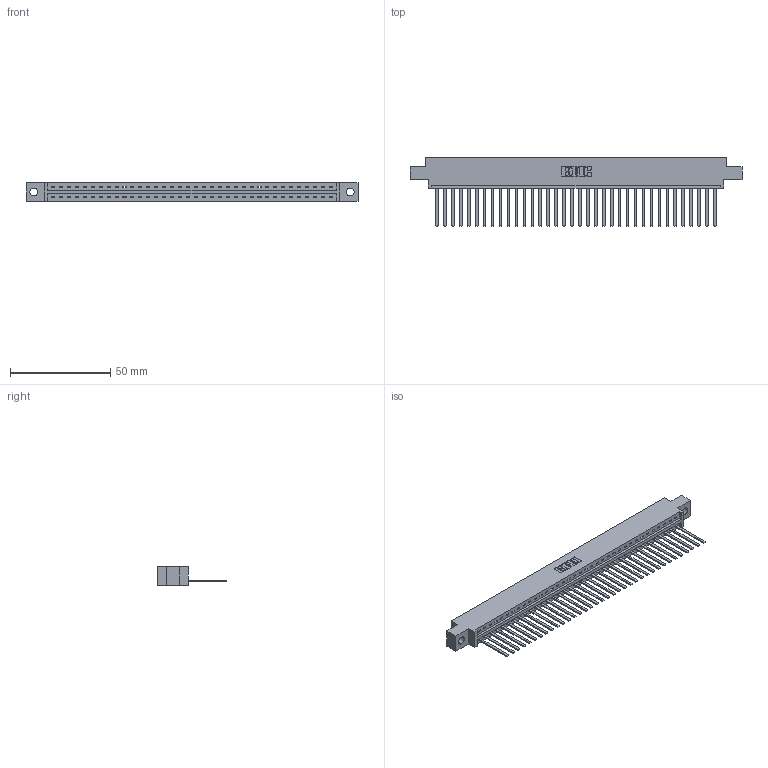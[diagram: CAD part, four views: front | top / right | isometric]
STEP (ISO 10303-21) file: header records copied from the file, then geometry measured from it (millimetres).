
FILE_DESCRIPTION (( 'STEP AP203' ), '1' );
FILE_NAME ('337-036-544-604.STEP', '2018-08-07T23:34:09', ( '' ), ( '' ), 'SwSTEP 2.0', 'SolidWorks 2016', '' );
FILE_SCHEMA (( 'CONFIG_CONTROL_DESIGN' ));
Length unit declared in the file: inch
Products named in the file (3): 345-292-001_345-293-144; 337-036-544-604; 337 Part_0.170 Offset - 0.156 Dia-TH
Assembly tree (37 placements, depth 2):
  337-036-544-604
    337 Part_0.170 Offset - 0.156 Dia-TH
    345-292-001_345-293-144  x36
Bounding box: 165.66 x 34.3 x 9.4 mm (x, y, z)
Volume: 17353.9 mm3; surface area: 19162.6 mm2
Topology: 37 solids, 37 shells, 2134 faces, 6443 edges, 4246 vertices
Faces by surface type: plane 1586, cylinder 548
Entity records: 27487 total; most frequent: CARTESIAN_POINT 4794, ORIENTED_EDGE 4766, DIRECTION 4043, EDGE_CURVE 2383, LINE 2259, VECTOR 2259, VERTEX_POINT 1586, AXIS2_PLACEMENT_3D 892
